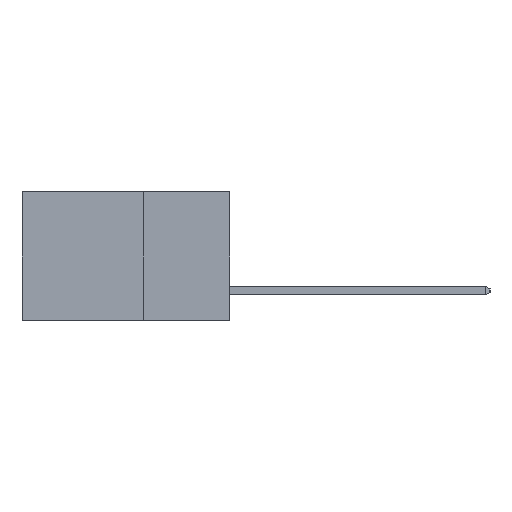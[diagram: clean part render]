
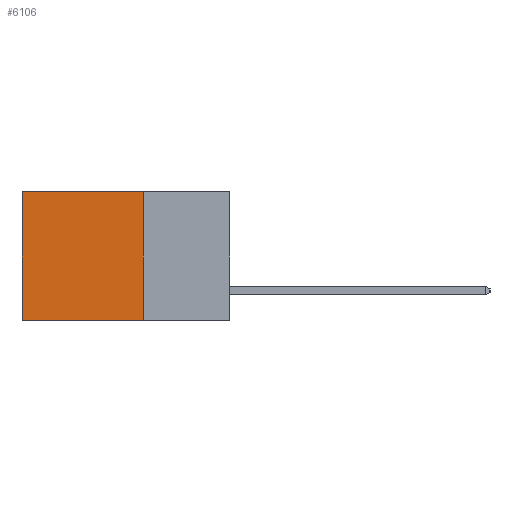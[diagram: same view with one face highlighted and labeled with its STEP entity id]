
A CAD part, left-side view. The second image highlights one B-rep face of the part: STEP entity #6106.
In plain terms, the highlighted planar face has unit normal (-1, 0, 0).
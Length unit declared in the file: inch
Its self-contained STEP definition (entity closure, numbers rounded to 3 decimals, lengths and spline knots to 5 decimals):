
#812 = EDGE_LOOP ( 'NONE', ( #10577, #7605, #3325, #12616 ) ) ;
#853 = VERTEX_POINT ( 'NONE', #13392 ) ;
#1424 = DIRECTION ( 'NONE',  ( 0., 1., 0. ) ) ;
#1464 = VECTOR ( 'NONE', #10069, 39.37008 ) ;
#2097 = CARTESIAN_POINT ( 'NONE',  ( 0.2615, 0.6, -0.37 ) ) ;
#2139 = DIRECTION ( 'NONE',  ( 0., 1., 0. ) ) ;
#2514 = CARTESIAN_POINT ( 'NONE',  ( 0.2615, 0.6, 0. ) ) ;
#2788 = LINE ( 'NONE', #13190, #10221 ) ;
#3174 = DIRECTION ( 'NONE',  ( 1., 0., 0. ) ) ;
#3303 = EDGE_CURVE ( 'NONE', #13236, #6093, #10452, .T. ) ;
#3325 = ORIENTED_EDGE ( 'NONE', *, *, #5898, .F. ) ;
#3450 = EDGE_CURVE ( 'NONE', #853, #9622, #9301, .T. ) ;
#4530 = VECTOR ( 'NONE', #2139, 39.37008 ) ;
#4976 = AXIS2_PLACEMENT_3D ( 'NONE', #9526, #3174, #12680 ) ;
#5577 = CARTESIAN_POINT ( 'NONE',  ( 0.2615, 0.25, -0.37 ) ) ;
#5750 = LINE ( 'NONE', #8824, #1464 ) ;
#5898 = EDGE_CURVE ( 'NONE', #853, #13236, #2788, .T. ) ;
#6093 = VERTEX_POINT ( 'NONE', #2097 ) ;
#6106 = ADVANCED_FACE ( 'NONE', ( #6886 ), #7483, .F. ) ;
#6362 = EDGE_CURVE ( 'NONE', #9622, #6093, #5750, .T. ) ;
#6886 = FACE_OUTER_BOUND ( 'NONE', #812, .T. ) ;
#7483 = PLANE ( 'NONE',  #4976 ) ;
#7605 = ORIENTED_EDGE ( 'NONE', *, *, #3303, .F. ) ;
#8824 = CARTESIAN_POINT ( 'NONE',  ( 0.2615, 0.6, -0.37 ) ) ;
#9301 = LINE ( 'NONE', #10490, #4530 ) ;
#9526 = CARTESIAN_POINT ( 'NONE',  ( 0.2615, 0.25, -0.37 ) ) ;
#9622 = VERTEX_POINT ( 'NONE', #2514 ) ;
#10069 = DIRECTION ( 'NONE',  ( 0., 0., -1. ) ) ;
#10221 = VECTOR ( 'NONE', #12215, 39.37008 ) ;
#10361 = CARTESIAN_POINT ( 'NONE',  ( 0.2615, 0.25, -0.37 ) ) ;
#10452 = LINE ( 'NONE', #5577, #11953 ) ;
#10490 = CARTESIAN_POINT ( 'NONE',  ( 0.2615, 0.25, 0. ) ) ;
#10577 = ORIENTED_EDGE ( 'NONE', *, *, #6362, .T. ) ;
#11953 = VECTOR ( 'NONE', #1424, 39.37008 ) ;
#12215 = DIRECTION ( 'NONE',  ( 0., 0., -1. ) ) ;
#12616 = ORIENTED_EDGE ( 'NONE', *, *, #3450, .T. ) ;
#12680 = DIRECTION ( 'NONE',  ( 0., 0., -1. ) ) ;
#13190 = CARTESIAN_POINT ( 'NONE',  ( 0.2615, 0.25, -0.37 ) ) ;
#13236 = VERTEX_POINT ( 'NONE', #10361 ) ;
#13392 = CARTESIAN_POINT ( 'NONE',  ( 0.2615, 0.25, 0. ) ) ;
